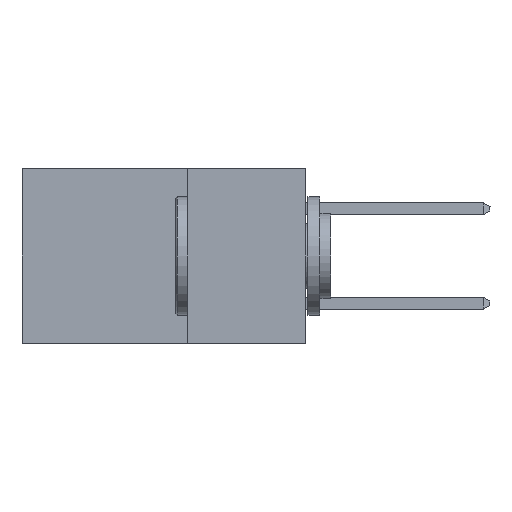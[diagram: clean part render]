
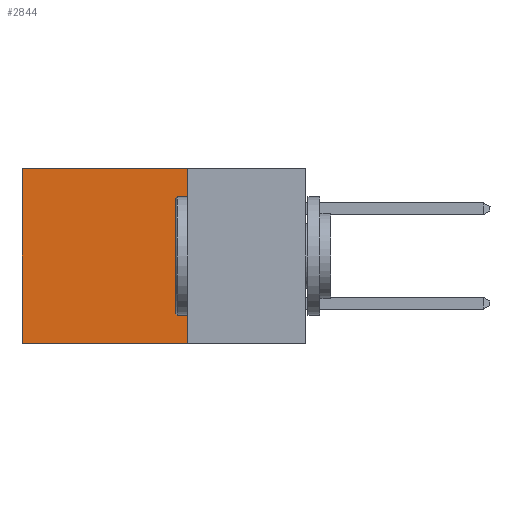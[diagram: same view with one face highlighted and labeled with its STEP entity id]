
A CAD part, left-side view. The second image highlights one B-rep face of the part: STEP entity #2844.
In plain terms, the highlighted planar face has unit normal (-1, 0, 0).
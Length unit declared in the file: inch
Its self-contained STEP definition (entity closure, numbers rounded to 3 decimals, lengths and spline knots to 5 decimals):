
#404 = CARTESIAN_POINT ( 'NONE',  ( 0.298, 0.25, 0. ) ) ;
#987 = ORIENTED_EDGE ( 'NONE', *, *, #17276, .T. ) ;
#1169 = CARTESIAN_POINT ( 'NONE',  ( 0.298, 0.25, -0.37 ) ) ;
#1365 = VECTOR ( 'NONE', #7230, 39.37008 ) ;
#1825 = LINE ( 'NONE', #5757, #1365 ) ;
#2097 = VERTEX_POINT ( 'NONE', #404 ) ;
#2130 = EDGE_CURVE ( 'NONE', #6833, #2510, #16513, .T. ) ;
#2510 = VERTEX_POINT ( 'NONE', #16410 ) ;
#2844 = ADVANCED_FACE ( 'NONE', ( #4419 ), #5652, .F. ) ;
#3647 = VERTEX_POINT ( 'NONE', #11188 ) ;
#4094 = LINE ( 'NONE', #15150, #15461 ) ;
#4419 = FACE_OUTER_BOUND ( 'NONE', #6246, .T. ) ;
#5136 = VECTOR ( 'NONE', #10043, 39.37008 ) ;
#5650 = DIRECTION ( 'NONE',  ( 1., 0., 0. ) ) ;
#5652 = PLANE ( 'NONE',  #17855 ) ;
#5684 = CARTESIAN_POINT ( 'NONE',  ( 0.298, 0.25, 0. ) ) ;
#5757 = CARTESIAN_POINT ( 'NONE',  ( 0.298, 0.25, 0. ) ) ;
#6218 = DIRECTION ( 'NONE',  ( 0., 0., -1. ) ) ;
#6246 = EDGE_LOOP ( 'NONE', ( #17290, #9235, #10101, #987 ) ) ;
#6791 = CARTESIAN_POINT ( 'NONE',  ( 0.298, 0.25, 0. ) ) ;
#6833 = VERTEX_POINT ( 'NONE', #1169 ) ;
#7230 = DIRECTION ( 'NONE',  ( 0., 1., 0. ) ) ;
#9235 = ORIENTED_EDGE ( 'NONE', *, *, #2130, .F. ) ;
#10043 = DIRECTION ( 'NONE',  ( 0., 1., 0. ) ) ;
#10101 = ORIENTED_EDGE ( 'NONE', *, *, #15324, .F. ) ;
#11188 = CARTESIAN_POINT ( 'NONE',  ( 0.298, 0.6, 0. ) ) ;
#11952 = LINE ( 'NONE', #5684, #15327 ) ;
#12379 = DIRECTION ( 'NONE',  ( 0., 0., -1. ) ) ;
#15150 = CARTESIAN_POINT ( 'NONE',  ( 0.298, 0.6, 0. ) ) ;
#15324 = EDGE_CURVE ( 'NONE', #2097, #6833, #11952, .T. ) ;
#15327 = VECTOR ( 'NONE', #17528, 39.37008 ) ;
#15461 = VECTOR ( 'NONE', #12379, 39.37008 ) ;
#15736 = CARTESIAN_POINT ( 'NONE',  ( 0.298, 0.25, -0.37 ) ) ;
#16410 = CARTESIAN_POINT ( 'NONE',  ( 0.298, 0.6, -0.37 ) ) ;
#16513 = LINE ( 'NONE', #15736, #5136 ) ;
#17276 = EDGE_CURVE ( 'NONE', #2097, #3647, #1825, .T. ) ;
#17290 = ORIENTED_EDGE ( 'NONE', *, *, #18853, .T. ) ;
#17528 = DIRECTION ( 'NONE',  ( 0., 0., -1. ) ) ;
#17855 = AXIS2_PLACEMENT_3D ( 'NONE', #6791, #5650, #6218 ) ;
#18853 = EDGE_CURVE ( 'NONE', #3647, #2510, #4094, .T. ) ;
